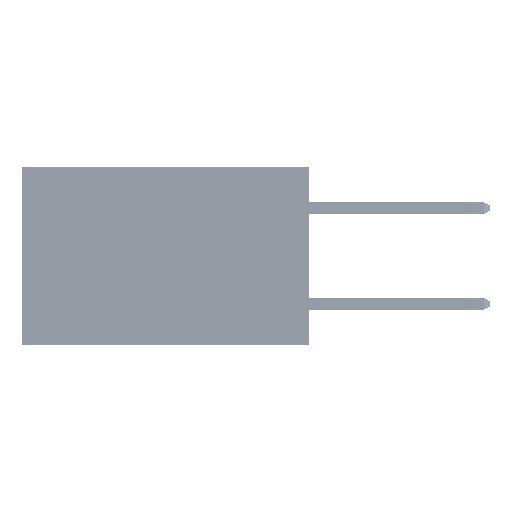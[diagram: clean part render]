
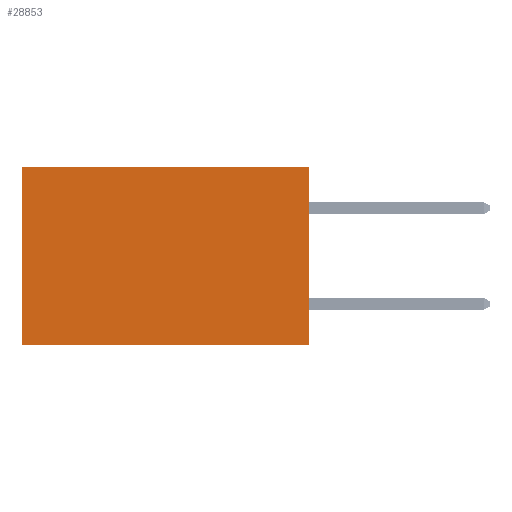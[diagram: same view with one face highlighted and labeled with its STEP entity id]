
A CAD part, left-side view. The second image highlights one B-rep face of the part: STEP entity #28853.
In plain terms, the highlighted planar face has unit normal (-1, 0, 0).
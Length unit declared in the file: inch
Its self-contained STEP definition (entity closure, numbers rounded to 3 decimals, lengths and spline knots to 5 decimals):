
#319 = LINE ( 'NONE', #41569, #30963 ) ;
#1377 = DIRECTION ( 'NONE',  ( 1., 0., 0. ) ) ;
#1729 = LINE ( 'NONE', #33811, #25003 ) ;
#2113 = VERTEX_POINT ( 'NONE', #25867 ) ;
#8075 = DIRECTION ( 'NONE',  ( 0., 0., -1. ) ) ;
#9048 = LINE ( 'NONE', #28500, #17582 ) ;
#11152 = CARTESIAN_POINT ( 'NONE',  ( 0.2875, 0.6, 0. ) ) ;
#11594 = ORIENTED_EDGE ( 'NONE', *, *, #42672, .T. ) ;
#12633 = PLANE ( 'NONE',  #27489 ) ;
#14332 = EDGE_CURVE ( 'NONE', #2113, #33102, #319, .T. ) ;
#16277 = CARTESIAN_POINT ( 'NONE',  ( 0.2875, 0., 0. ) ) ;
#16459 = VERTEX_POINT ( 'NONE', #46731 ) ;
#17582 = VECTOR ( 'NONE', #39036, 39.37008 ) ;
#17974 = ORIENTED_EDGE ( 'NONE', *, *, #14332, .F. ) ;
#21097 = LINE ( 'NONE', #40921, #39338 ) ;
#23724 = DIRECTION ( 'NONE',  ( 0., 0., -1. ) ) ;
#25003 = VECTOR ( 'NONE', #8075, 39.37008 ) ;
#25867 = CARTESIAN_POINT ( 'NONE',  ( 0.2875, 0., -0.37 ) ) ;
#26513 = EDGE_LOOP ( 'NONE', ( #39134, #17974, #31640, #11594 ) ) ;
#27387 = FACE_OUTER_BOUND ( 'NONE', #26513, .T. ) ;
#27489 = AXIS2_PLACEMENT_3D ( 'NONE', #16277, #1377, #23724 ) ;
#28500 = CARTESIAN_POINT ( 'NONE',  ( 0.2875, 0., 0. ) ) ;
#28853 = ADVANCED_FACE ( 'NONE', ( #27387 ), #12633, .F. ) ;
#29745 = EDGE_CURVE ( 'NONE', #16459, #2113, #1729, .T. ) ;
#30963 = VECTOR ( 'NONE', #41734, 39.37008 ) ;
#31640 = ORIENTED_EDGE ( 'NONE', *, *, #29745, .F. ) ;
#33102 = VERTEX_POINT ( 'NONE', #38833 ) ;
#33811 = CARTESIAN_POINT ( 'NONE',  ( 0.2875, 0., 0. ) ) ;
#34844 = VERTEX_POINT ( 'NONE', #11152 ) ;
#35494 = EDGE_CURVE ( 'NONE', #34844, #33102, #21097, .T. ) ;
#38833 = CARTESIAN_POINT ( 'NONE',  ( 0.2875, 0.6, -0.37 ) ) ;
#39036 = DIRECTION ( 'NONE',  ( 0., 1., 0. ) ) ;
#39134 = ORIENTED_EDGE ( 'NONE', *, *, #35494, .T. ) ;
#39338 = VECTOR ( 'NONE', #44584, 39.37008 ) ;
#40921 = CARTESIAN_POINT ( 'NONE',  ( 0.2875, 0.6, 0. ) ) ;
#41569 = CARTESIAN_POINT ( 'NONE',  ( 0.2875, 0., -0.37 ) ) ;
#41734 = DIRECTION ( 'NONE',  ( 0., 1., 0. ) ) ;
#42672 = EDGE_CURVE ( 'NONE', #16459, #34844, #9048, .T. ) ;
#44584 = DIRECTION ( 'NONE',  ( 0., 0., -1. ) ) ;
#46731 = CARTESIAN_POINT ( 'NONE',  ( 0.2875, 0., 0. ) ) ;
